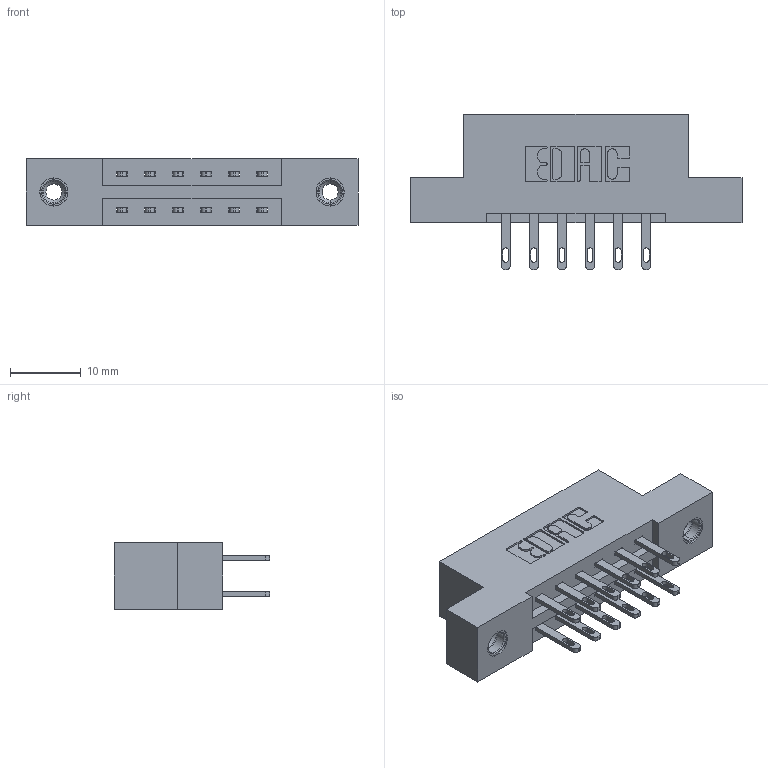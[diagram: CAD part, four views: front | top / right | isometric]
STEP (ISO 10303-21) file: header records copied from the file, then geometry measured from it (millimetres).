
FILE_DESCRIPTION (( 'STEP AP203' ), '1' );
FILE_NAME ('887-012-500-208.STEP', '2020-09-20T16:23:42', ( '' ), ( '' ), 'SwSTEP 2.0', 'SolidWorks 2020', '' );
FILE_SCHEMA (( 'CONFIG_CONTROL_DESIGN' ));
Length unit declared in the file: inch
Products named in the file (4): 345-292-001_345-293-100; 837 Part_Flush Mounting Lugs - 0.156 Dia-TI; 345-250-001_345-250-003-102; 887-012-500-208
Assembly tree (15 placements, depth 2):
  887-012-500-208
    837 Part_Flush Mounting Lugs - 0.156 Dia-TI
    345-292-001_345-293-100  x12
    345-250-001_345-250-003-102  x2
Bounding box: 46.79 x 21.85 x 9.4 mm (x, y, z)
Volume: 4481.7 mm3; surface area: 4874 mm2
Topology: 15 solids, 15 shells, 774 faces, 2283 edges, 1514 vertices
Faces by surface type: plane 486, cylinder 272, cone 12, torus 4
Entity records: 10424 total; most frequent: CARTESIAN_POINT 1765, ORIENTED_EDGE 1694, DIRECTION 1601, EDGE_CURVE 847, LINE 695, VECTOR 695, VERTEX_POINT 560, AXIS2_PLACEMENT_3D 453
